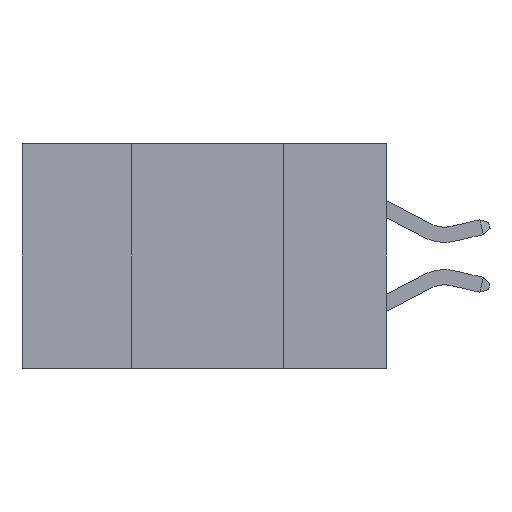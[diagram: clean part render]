
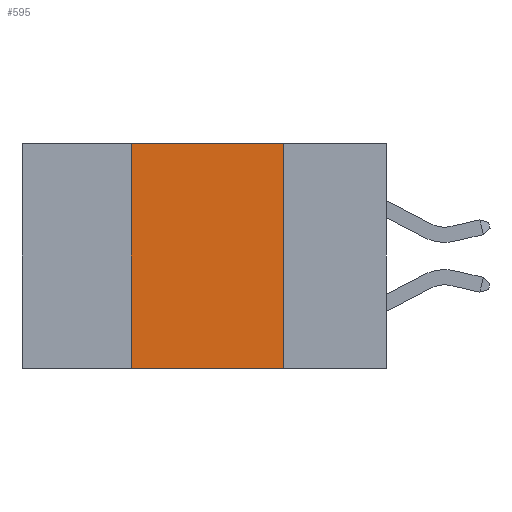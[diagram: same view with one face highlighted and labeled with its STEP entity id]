
A CAD part, left-side view. The second image highlights one B-rep face of the part: STEP entity #595.
In plain terms, the highlighted planar face has unit normal (-1, 0, 0).
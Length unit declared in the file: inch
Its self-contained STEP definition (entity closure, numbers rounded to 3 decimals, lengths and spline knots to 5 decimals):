
#595 = ADVANCED_FACE ( 'NONE', ( #22053 ), #4839, .F. ) ;
#686 = DIRECTION ( 'NONE',  ( 0., -1., 0. ) ) ;
#2618 = LINE ( 'NONE', #16590, #19238 ) ;
#2868 = VECTOR ( 'NONE', #19690, 39.37008 ) ;
#2901 = DIRECTION ( 'NONE',  ( 1., 0., 0. ) ) ;
#4839 = PLANE ( 'NONE',  #24880 ) ;
#5298 = VERTEX_POINT ( 'NONE', #19918 ) ;
#5916 = CARTESIAN_POINT ( 'NONE',  ( 0., 0.42, 0. ) ) ;
#7629 = DIRECTION ( 'NONE',  ( 0., 0., -1. ) ) ;
#8865 = EDGE_LOOP ( 'NONE', ( #21128, #24990, #24928, #10972 ) ) ;
#9572 = CARTESIAN_POINT ( 'NONE',  ( 0., 0.6, -0.37 ) ) ;
#10972 = ORIENTED_EDGE ( 'NONE', *, *, #21297, .T. ) ;
#11309 = EDGE_CURVE ( 'NONE', #23228, #12077, #2618, .T. ) ;
#12077 = VERTEX_POINT ( 'NONE', #16282 ) ;
#12718 = CARTESIAN_POINT ( 'NONE',  ( 0., 0.6, 0. ) ) ;
#13856 = CARTESIAN_POINT ( 'NONE',  ( 0., 0.17, -0.37 ) ) ;
#14159 = DIRECTION ( 'NONE',  ( 0., 0., -1. ) ) ;
#14368 = DIRECTION ( 'NONE',  ( 0., 0., 1. ) ) ;
#14706 = VERTEX_POINT ( 'NONE', #18592 ) ;
#15280 = LINE ( 'NONE', #13856, #19842 ) ;
#16282 = CARTESIAN_POINT ( 'NONE',  ( 0., 0.17, 0. ) ) ;
#16504 = VECTOR ( 'NONE', #14368, 39.37008 ) ;
#16590 = CARTESIAN_POINT ( 'NONE',  ( 0., 0.6, 0. ) ) ;
#17624 = LINE ( 'NONE', #9572, #2868 ) ;
#18013 = LINE ( 'NONE', #23935, #16504 ) ;
#18592 = CARTESIAN_POINT ( 'NONE',  ( 0., 0.42, -0.37 ) ) ;
#19238 = VECTOR ( 'NONE', #686, 39.37008 ) ;
#19690 = DIRECTION ( 'NONE',  ( 0., -1., 0. ) ) ;
#19842 = VECTOR ( 'NONE', #7629, 39.37008 ) ;
#19918 = CARTESIAN_POINT ( 'NONE',  ( 0., 0.17, -0.37 ) ) ;
#21128 = ORIENTED_EDGE ( 'NONE', *, *, #22686, .F. ) ;
#21297 = EDGE_CURVE ( 'NONE', #14706, #5298, #17624, .T. ) ;
#21438 = EDGE_CURVE ( 'NONE', #14706, #23228, #18013, .T. ) ;
#22053 = FACE_OUTER_BOUND ( 'NONE', #8865, .T. ) ;
#22686 = EDGE_CURVE ( 'NONE', #12077, #5298, #15280, .T. ) ;
#23228 = VERTEX_POINT ( 'NONE', #5916 ) ;
#23935 = CARTESIAN_POINT ( 'NONE',  ( 0., 0.42, -0.37 ) ) ;
#24880 = AXIS2_PLACEMENT_3D ( 'NONE', #12718, #2901, #14159 ) ;
#24928 = ORIENTED_EDGE ( 'NONE', *, *, #21438, .F. ) ;
#24990 = ORIENTED_EDGE ( 'NONE', *, *, #11309, .F. ) ;
